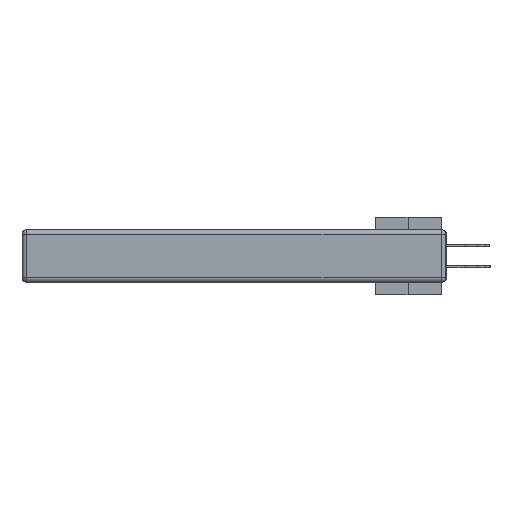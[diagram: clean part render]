
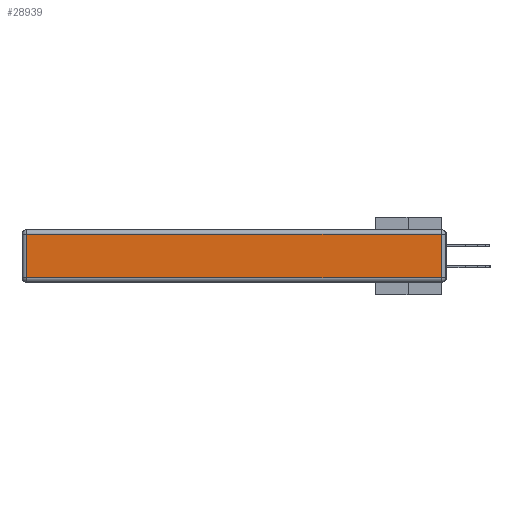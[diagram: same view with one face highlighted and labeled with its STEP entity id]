
A CAD part, left-side view. The second image highlights one B-rep face of the part: STEP entity #28939.
In plain terms, the highlighted planar face has unit normal (-1, 0, 0).
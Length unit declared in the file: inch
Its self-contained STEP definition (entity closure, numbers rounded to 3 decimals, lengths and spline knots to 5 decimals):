
#73 = PLANE ( 'NONE',  #22730 ) ;
#1710 = DIRECTION ( 'NONE',  ( 0., 0., 1. ) ) ;
#2029 = EDGE_CURVE ( 'NONE', #7953, #13940, #35760, .T. ) ;
#6318 = CARTESIAN_POINT ( 'NONE',  ( 0., 2.72, -0.03 ) ) ;
#7953 = VERTEX_POINT ( 'NONE', #24129 ) ;
#8425 = EDGE_CURVE ( 'NONE', #13940, #19162, #17566, .T. ) ;
#8598 = VERTEX_POINT ( 'NONE', #30522 ) ;
#8859 = VECTOR ( 'NONE', #17286, 39.37008 ) ;
#10830 = FACE_OUTER_BOUND ( 'NONE', #25837, .T. ) ;
#10858 = CARTESIAN_POINT ( 'NONE',  ( 0., 2.72, -0.343 ) ) ;
#11291 = ORIENTED_EDGE ( 'NONE', *, *, #15181, .T. ) ;
#12718 = LINE ( 'NONE', #31269, #17103 ) ;
#13640 = CARTESIAN_POINT ( 'NONE',  ( 0., 0., -0.313 ) ) ;
#13940 = VERTEX_POINT ( 'NONE', #6318 ) ;
#15181 = EDGE_CURVE ( 'NONE', #8598, #7953, #12718, .T. ) ;
#16795 = DIRECTION ( 'NONE',  ( 0., -1., 0. ) ) ;
#17103 = VECTOR ( 'NONE', #34948, 39.37008 ) ;
#17286 = DIRECTION ( 'NONE',  ( 0., 1., 0. ) ) ;
#17407 = VECTOR ( 'NONE', #16795, 39.37008 ) ;
#17447 = DIRECTION ( 'NONE',  ( 0., 0., -1. ) ) ;
#17566 = LINE ( 'NONE', #10858, #23879 ) ;
#19050 = ORIENTED_EDGE ( 'NONE', *, *, #32281, .T. ) ;
#19162 = VERTEX_POINT ( 'NONE', #19731 ) ;
#19731 = CARTESIAN_POINT ( 'NONE',  ( 0., 2.72, -0.313 ) ) ;
#22003 = CARTESIAN_POINT ( 'NONE',  ( 0., 0., -0.343 ) ) ;
#22244 = ORIENTED_EDGE ( 'NONE', *, *, #8425, .T. ) ;
#22730 = AXIS2_PLACEMENT_3D ( 'NONE', #22003, #30771, #1710 ) ;
#23879 = VECTOR ( 'NONE', #17447, 39.37008 ) ;
#24129 = CARTESIAN_POINT ( 'NONE',  ( 0., 0.03, -0.03 ) ) ;
#25837 = EDGE_LOOP ( 'NONE', ( #19050, #11291, #29015, #22244 ) ) ;
#28939 = ADVANCED_FACE ( 'NONE', ( #10830 ), #73, .T. ) ;
#29015 = ORIENTED_EDGE ( 'NONE', *, *, #2029, .T. ) ;
#30522 = CARTESIAN_POINT ( 'NONE',  ( 0., 0.03, -0.313 ) ) ;
#30771 = DIRECTION ( 'NONE',  ( -1., 0., 0. ) ) ;
#31269 = CARTESIAN_POINT ( 'NONE',  ( 0., 0.03, -0.343 ) ) ;
#32281 = EDGE_CURVE ( 'NONE', #19162, #8598, #35450, .T. ) ;
#34948 = DIRECTION ( 'NONE',  ( 0., 0., 1. ) ) ;
#35450 = LINE ( 'NONE', #13640, #17407 ) ;
#35760 = LINE ( 'NONE', #39009, #8859 ) ;
#39009 = CARTESIAN_POINT ( 'NONE',  ( 0., 2.75, -0.03 ) ) ;
